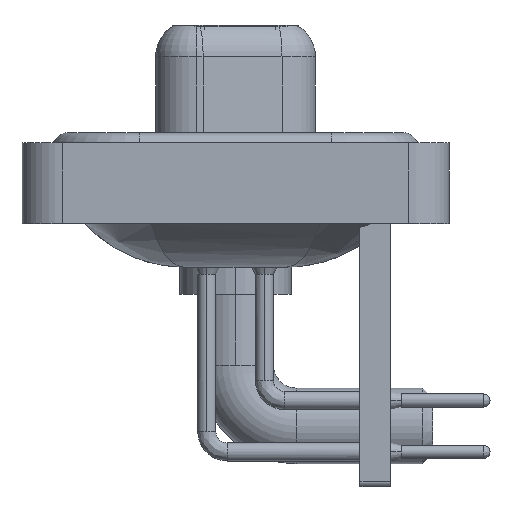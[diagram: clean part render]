
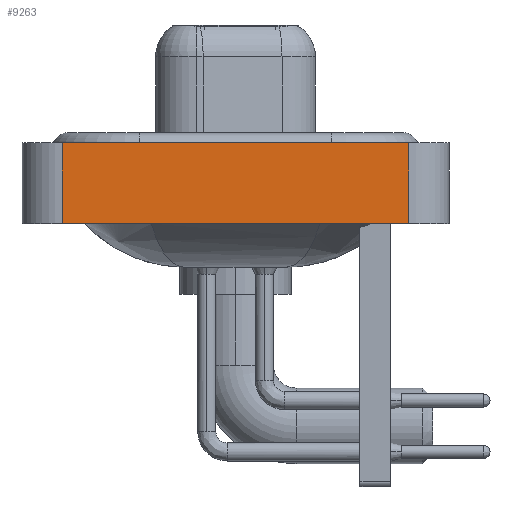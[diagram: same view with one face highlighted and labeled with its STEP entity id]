
A CAD part, left-side view. The second image highlights one B-rep face of the part: STEP entity #9263.
In plain terms, the highlighted planar face has unit normal (-1, 0, 0).
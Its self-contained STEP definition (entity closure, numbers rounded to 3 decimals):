
#1140 = VERTEX_POINT ( 'NONE', #16483 ) ;
#1741 = ORIENTED_EDGE ( 'NONE', *, *, #5735, .T. ) ;
#3246 = ORIENTED_EDGE ( 'NONE', *, *, #10944, .F. ) ;
#3320 = LINE ( 'NONE', #21308, #15572 ) ;
#3483 = CARTESIAN_POINT ( 'NONE',  ( -7.3, 8.55, -3.6 ) ) ;
#4041 = LINE ( 'NONE', #12847, #7097 ) ;
#4628 = DIRECTION ( 'NONE',  ( 0., 0., 1. ) ) ;
#4984 = DIRECTION ( 'NONE',  ( -1., 0., 0. ) ) ;
#5735 = EDGE_CURVE ( 'NONE', #22638, #15812, #4041, .T. ) ;
#6008 = EDGE_CURVE ( 'NONE', #22638, #1140, #3320, .T. ) ;
#6617 = CARTESIAN_POINT ( 'NONE',  ( -7.3, -8.55, -3.6 ) ) ;
#7086 = PLANE ( 'NONE',  #17565 ) ;
#7097 = VECTOR ( 'NONE', #20027, 1000. ) ;
#7268 = CARTESIAN_POINT ( 'NONE',  ( -7.3, -8.55, -3.6 ) ) ;
#9149 = DIRECTION ( 'NONE',  ( 0., -1., 0. ) ) ;
#9263 = ADVANCED_FACE ( 'NONE', ( #13893 ), #7086, .T. ) ;
#10492 = DIRECTION ( 'NONE',  ( 0., 0., 1. ) ) ;
#10914 = CARTESIAN_POINT ( 'NONE',  ( -7.3, -8.55, 0.4 ) ) ;
#10944 = EDGE_CURVE ( 'NONE', #1140, #13247, #19845, .T. ) ;
#12636 = VECTOR ( 'NONE', #9149, 1000. ) ;
#12847 = CARTESIAN_POINT ( 'NONE',  ( -7.3, -8.55, -3.6 ) ) ;
#13039 = EDGE_CURVE ( 'NONE', #15812, #13247, #13534, .T. ) ;
#13247 = VERTEX_POINT ( 'NONE', #21301 ) ;
#13534 = LINE ( 'NONE', #20719, #21787 ) ;
#13893 = FACE_OUTER_BOUND ( 'NONE', #18863, .T. ) ;
#14125 = DIRECTION ( 'NONE',  ( 0., 0., 1. ) ) ;
#15572 = VECTOR ( 'NONE', #10492, 1000. ) ;
#15812 = VERTEX_POINT ( 'NONE', #7268 ) ;
#16433 = ORIENTED_EDGE ( 'NONE', *, *, #13039, .T. ) ;
#16483 = CARTESIAN_POINT ( 'NONE',  ( -7.3, 8.55, 0.4 ) ) ;
#17565 = AXIS2_PLACEMENT_3D ( 'NONE', #6617, #4984, #14125 ) ;
#18863 = EDGE_LOOP ( 'NONE', ( #16433, #3246, #21895, #1741 ) ) ;
#19845 = LINE ( 'NONE', #10914, #12636 ) ;
#20027 = DIRECTION ( 'NONE',  ( 0., -1., 0. ) ) ;
#20719 = CARTESIAN_POINT ( 'NONE',  ( -7.3, -8.55, -3.6 ) ) ;
#21301 = CARTESIAN_POINT ( 'NONE',  ( -7.3, -8.55, 0.4 ) ) ;
#21308 = CARTESIAN_POINT ( 'NONE',  ( -7.3, 8.55, -3.6 ) ) ;
#21787 = VECTOR ( 'NONE', #4628, 1000. ) ;
#21895 = ORIENTED_EDGE ( 'NONE', *, *, #6008, .F. ) ;
#22638 = VERTEX_POINT ( 'NONE', #3483 ) ;
